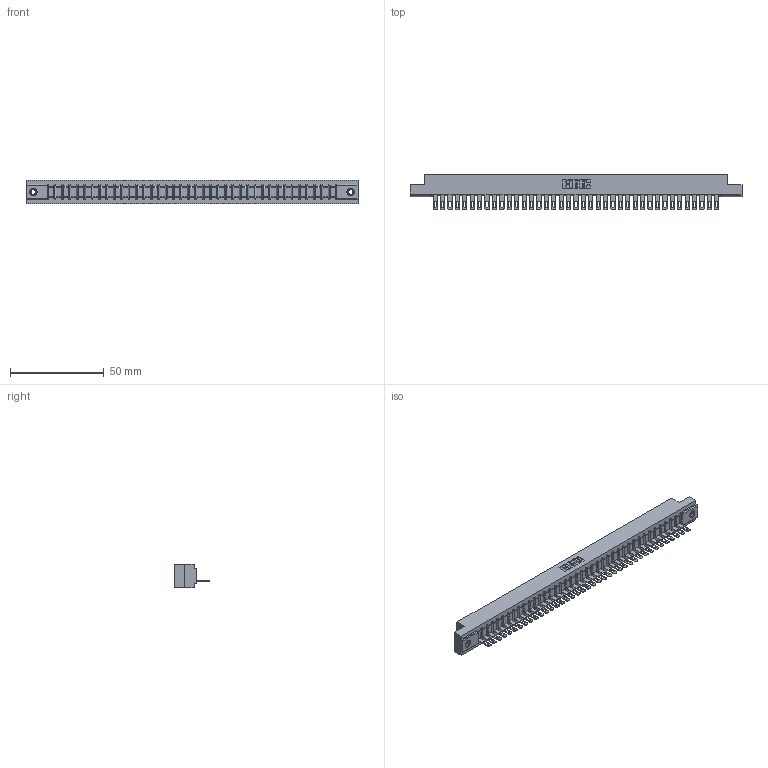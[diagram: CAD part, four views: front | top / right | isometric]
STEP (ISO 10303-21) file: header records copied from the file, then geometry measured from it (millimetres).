
FILE_DESCRIPTION (( 'STEP AP203' ), '1' );
FILE_NAME ('357-039-505-107.STEP', '2018-08-10T10:36:59', ( '' ), ( '' ), 'SwSTEP 2.0', 'SolidWorks 2016', '' );
FILE_SCHEMA (( 'CONFIG_CONTROL_DESIGN' ));
Length unit declared in the file: inch
Products named in the file (4): 307 Part_.156 Dia Mounting Holes; 307-290-001_505; 345-250-001_345-250-005-103; 357-039-505-107
Assembly tree (42 placements, depth 2):
  357-039-505-107
    307 Part_.156 Dia Mounting Holes
    307-290-001_505  x39
    345-250-001_345-250-005-103  x2
Bounding box: 177.55 x 19.18 x 12.7 mm (x, y, z)
Volume: 18453.7 mm3; surface area: 19869.3 mm2
Topology: 42 solids, 42 shells, 2402 faces, 6777 edges, 4350 vertices
Faces by surface type: plane 1506, cylinder 800, sphere 80, cone 12, torus 4
Entity records: 34963 total; most frequent: CARTESIAN_POINT 5867, ORIENTED_EDGE 5846, DIRECTION 5719, EDGE_CURVE 2923, VECTOR 2239, LINE 2239, VERTEX_POINT 1888, AXIS2_PLACEMENT_3D 1740
